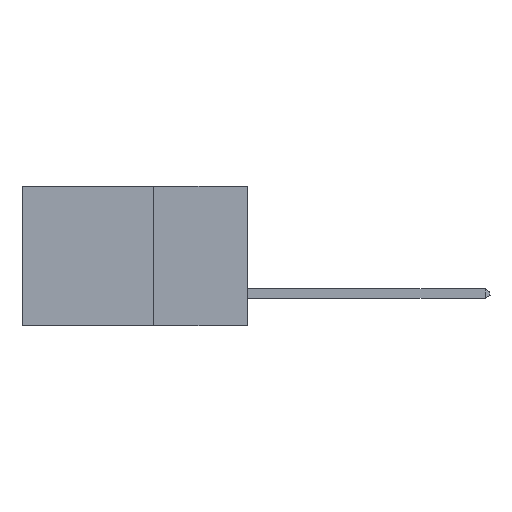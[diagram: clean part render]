
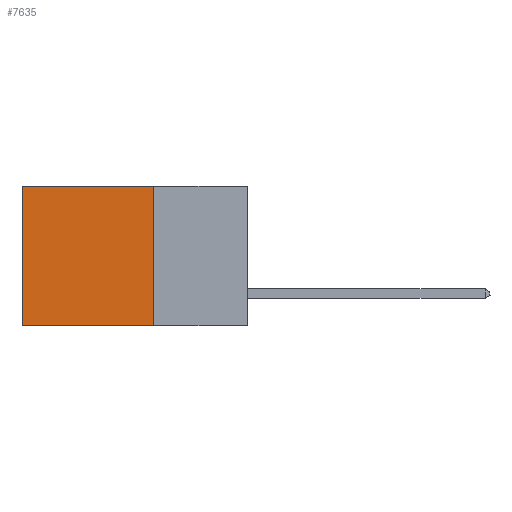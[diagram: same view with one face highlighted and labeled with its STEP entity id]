
A CAD part, left-side view. The second image highlights one B-rep face of the part: STEP entity #7635.
In plain terms, the highlighted planar face has unit normal (-1, 0, 0).
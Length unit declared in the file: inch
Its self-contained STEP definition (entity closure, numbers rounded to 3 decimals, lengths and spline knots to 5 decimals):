
#85 = CARTESIAN_POINT ( 'NONE',  ( 0.298, 0.25, 0. ) ) ;
#253 = EDGE_CURVE ( 'NONE', #5947, #9783, #9124, .T. ) ;
#1520 = VECTOR ( 'NONE', #12562, 39.37008 ) ;
#2811 = VECTOR ( 'NONE', #10716, 39.37008 ) ;
#3118 = VECTOR ( 'NONE', #3309, 39.37008 ) ;
#3309 = DIRECTION ( 'NONE',  ( 0., 1., 0. ) ) ;
#3642 = EDGE_CURVE ( 'NONE', #13312, #9783, #5455, .T. ) ;
#3925 = ORIENTED_EDGE ( 'NONE', *, *, #9921, .F. ) ;
#4961 = CARTESIAN_POINT ( 'NONE',  ( 0.298, 0.6, 0. ) ) ;
#5455 = LINE ( 'NONE', #15347, #1520 ) ;
#5667 = ORIENTED_EDGE ( 'NONE', *, *, #13203, .T. ) ;
#5947 = VERTEX_POINT ( 'NONE', #12520 ) ;
#6280 = LINE ( 'NONE', #13335, #2811 ) ;
#6360 = CARTESIAN_POINT ( 'NONE',  ( 0.298, 0.25, 0. ) ) ;
#6396 = PLANE ( 'NONE',  #14629 ) ;
#6454 = DIRECTION ( 'NONE',  ( 1., 0., 0. ) ) ;
#6749 = DIRECTION ( 'NONE',  ( 0., 1., 0. ) ) ;
#6842 = EDGE_LOOP ( 'NONE', ( #7186, #10749, #3925, #5667 ) ) ;
#7186 = ORIENTED_EDGE ( 'NONE', *, *, #3642, .T. ) ;
#7320 = CARTESIAN_POINT ( 'NONE',  ( 0.298, 0.25, 0. ) ) ;
#7635 = ADVANCED_FACE ( 'NONE', ( #8236 ), #6396, .F. ) ;
#8141 = CARTESIAN_POINT ( 'NONE',  ( 0.298, 0.25, -0.37 ) ) ;
#8236 = FACE_OUTER_BOUND ( 'NONE', #6842, .T. ) ;
#9124 = LINE ( 'NONE', #8141, #10973 ) ;
#9783 = VERTEX_POINT ( 'NONE', #13831 ) ;
#9921 = EDGE_CURVE ( 'NONE', #10775, #5947, #6280, .T. ) ;
#10353 = LINE ( 'NONE', #7320, #3118 ) ;
#10556 = DIRECTION ( 'NONE',  ( 0., 0., -1. ) ) ;
#10716 = DIRECTION ( 'NONE',  ( 0., 0., -1. ) ) ;
#10749 = ORIENTED_EDGE ( 'NONE', *, *, #253, .F. ) ;
#10775 = VERTEX_POINT ( 'NONE', #6360 ) ;
#10973 = VECTOR ( 'NONE', #6749, 39.37008 ) ;
#12520 = CARTESIAN_POINT ( 'NONE',  ( 0.298, 0.25, -0.37 ) ) ;
#12562 = DIRECTION ( 'NONE',  ( 0., 0., -1. ) ) ;
#13203 = EDGE_CURVE ( 'NONE', #10775, #13312, #10353, .T. ) ;
#13312 = VERTEX_POINT ( 'NONE', #4961 ) ;
#13335 = CARTESIAN_POINT ( 'NONE',  ( 0.298, 0.25, 0. ) ) ;
#13831 = CARTESIAN_POINT ( 'NONE',  ( 0.298, 0.6, -0.37 ) ) ;
#14629 = AXIS2_PLACEMENT_3D ( 'NONE', #85, #6454, #10556 ) ;
#15347 = CARTESIAN_POINT ( 'NONE',  ( 0.298, 0.6, 0. ) ) ;
